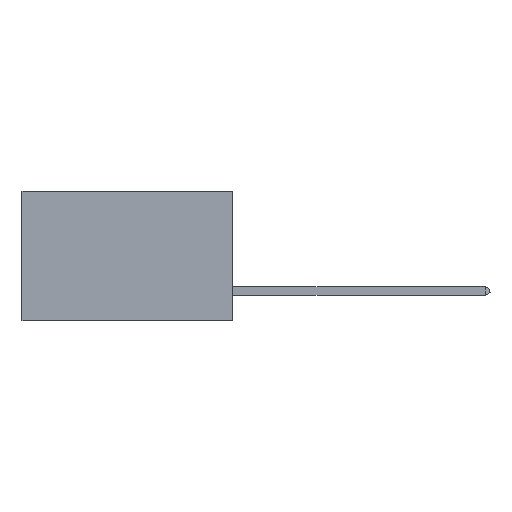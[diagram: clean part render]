
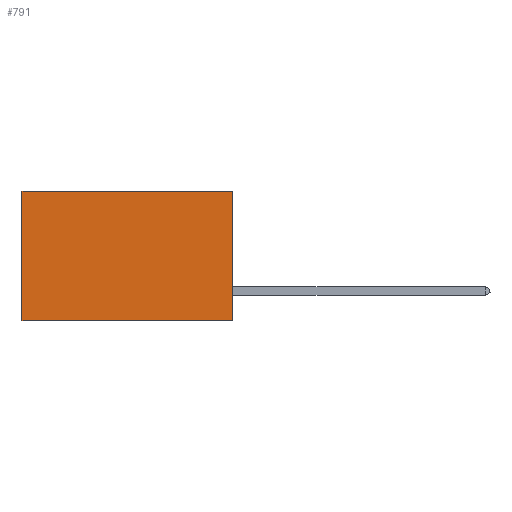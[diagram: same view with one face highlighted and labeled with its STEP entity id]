
A CAD part, left-side view. The second image highlights one B-rep face of the part: STEP entity #791.
In plain terms, the highlighted planar face has unit normal (-1, 0, 0).
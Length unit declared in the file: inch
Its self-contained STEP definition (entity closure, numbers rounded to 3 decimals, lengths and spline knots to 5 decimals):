
#791 = ADVANCED_FACE ( 'NONE', ( #9232 ), #19256, .F. ) ;
#2485 = LINE ( 'NONE', #27895, #30411 ) ;
#3283 = AXIS2_PLACEMENT_3D ( 'NONE', #32607, #16410, #19142 ) ;
#6485 = LINE ( 'NONE', #18689, #21677 ) ;
#7590 = ORIENTED_EDGE ( 'NONE', *, *, #24685, .F. ) ;
#7612 = VECTOR ( 'NONE', #20729, 39.37008 ) ;
#9232 = FACE_OUTER_BOUND ( 'NONE', #23968, .T. ) ;
#10189 = ORIENTED_EDGE ( 'NONE', *, *, #24386, .F. ) ;
#10515 = EDGE_CURVE ( 'NONE', #18703, #23002, #2485, .T. ) ;
#11150 = CARTESIAN_POINT ( 'NONE',  ( 0.2875, 0., 0. ) ) ;
#12752 = CARTESIAN_POINT ( 'NONE',  ( 0.2875, 0., 0. ) ) ;
#15197 = ORIENTED_EDGE ( 'NONE', *, *, #10515, .T. ) ;
#16240 = EDGE_CURVE ( 'NONE', #23002, #32443, #6485, .T. ) ;
#16372 = CARTESIAN_POINT ( 'NONE',  ( 0.2875, 0.6, -0.37 ) ) ;
#16410 = DIRECTION ( 'NONE',  ( 1., 0., 0. ) ) ;
#18689 = CARTESIAN_POINT ( 'NONE',  ( 0.2875, 0.6, 0. ) ) ;
#18703 = VERTEX_POINT ( 'NONE', #12752 ) ;
#19142 = DIRECTION ( 'NONE',  ( 0., 0., -1. ) ) ;
#19256 = PLANE ( 'NONE',  #3283 ) ;
#19456 = VECTOR ( 'NONE', #19461, 39.37008 ) ;
#19461 = DIRECTION ( 'NONE',  ( 0., 0., -1. ) ) ;
#19709 = DIRECTION ( 'NONE',  ( 0., 1., 0. ) ) ;
#20729 = DIRECTION ( 'NONE',  ( 0., 1., 0. ) ) ;
#21677 = VECTOR ( 'NONE', #29547, 39.37008 ) ;
#22417 = LINE ( 'NONE', #11150, #19456 ) ;
#23002 = VERTEX_POINT ( 'NONE', #27088 ) ;
#23968 = EDGE_LOOP ( 'NONE', ( #26865, #7590, #10189, #15197 ) ) ;
#24092 = VERTEX_POINT ( 'NONE', #31667 ) ;
#24386 = EDGE_CURVE ( 'NONE', #18703, #24092, #22417, .T. ) ;
#24685 = EDGE_CURVE ( 'NONE', #24092, #32443, #27460, .T. ) ;
#26865 = ORIENTED_EDGE ( 'NONE', *, *, #16240, .T. ) ;
#27088 = CARTESIAN_POINT ( 'NONE',  ( 0.2875, 0.6, 0. ) ) ;
#27460 = LINE ( 'NONE', #34114, #7612 ) ;
#27895 = CARTESIAN_POINT ( 'NONE',  ( 0.2875, 0., 0. ) ) ;
#29547 = DIRECTION ( 'NONE',  ( 0., 0., -1. ) ) ;
#30411 = VECTOR ( 'NONE', #19709, 39.37008 ) ;
#31667 = CARTESIAN_POINT ( 'NONE',  ( 0.2875, 0., -0.37 ) ) ;
#32443 = VERTEX_POINT ( 'NONE', #16372 ) ;
#32607 = CARTESIAN_POINT ( 'NONE',  ( 0.2875, 0., 0. ) ) ;
#34114 = CARTESIAN_POINT ( 'NONE',  ( 0.2875, 0., -0.37 ) ) ;
